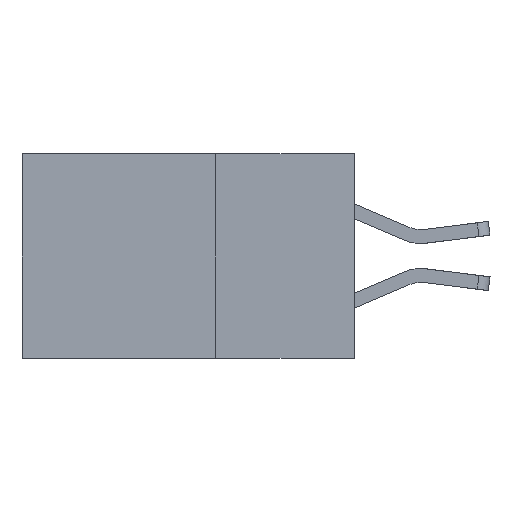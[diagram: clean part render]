
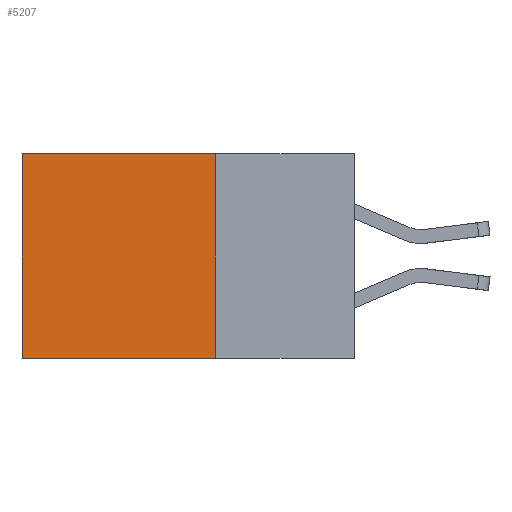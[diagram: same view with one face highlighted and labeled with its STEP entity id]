
A CAD part, left-side view. The second image highlights one B-rep face of the part: STEP entity #5207.
In plain terms, the highlighted planar face has unit normal (-1, 0, 0).
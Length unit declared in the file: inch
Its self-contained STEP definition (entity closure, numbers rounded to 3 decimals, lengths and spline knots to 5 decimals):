
#94 = EDGE_CURVE ( 'NONE', #6212, #6668, #8114, .T. ) ;
#167 = LINE ( 'NONE', #8510, #6126 ) ;
#256 = VERTEX_POINT ( 'NONE', #7802 ) ;
#273 = ORIENTED_EDGE ( 'NONE', *, *, #2507, .T. ) ;
#386 = ORIENTED_EDGE ( 'NONE', *, *, #94, .F. ) ;
#502 = VERTEX_POINT ( 'NONE', #7312 ) ;
#511 = ORIENTED_EDGE ( 'NONE', *, *, #9376, .F. ) ;
#541 = DIRECTION ( 'NONE',  ( 1., 0., 0. ) ) ;
#648 = DIRECTION ( 'NONE',  ( 0., 0., -1. ) ) ;
#697 = CARTESIAN_POINT ( 'NONE',  ( 0.2615, 0.25, -0.37 ) ) ;
#748 = PLANE ( 'NONE',  #6104 ) ;
#918 = VECTOR ( 'NONE', #7294, 39.37008 ) ;
#974 = ORIENTED_EDGE ( 'NONE', *, *, #1633, .T. ) ;
#1185 = LINE ( 'NONE', #9366, #918 ) ;
#1633 = EDGE_CURVE ( 'NONE', #256, #502, #167, .T. ) ;
#1640 = DIRECTION ( 'NONE',  ( 0., 0., -1. ) ) ;
#1772 = EDGE_LOOP ( 'NONE', ( #273, #386, #511, #974 ) ) ;
#2507 = EDGE_CURVE ( 'NONE', #502, #6668, #1185, .T. ) ;
#2547 = CARTESIAN_POINT ( 'NONE',  ( 0.2615, 0.6, -0.37 ) ) ;
#2885 = VECTOR ( 'NONE', #2998, 39.37008 ) ;
#2998 = DIRECTION ( 'NONE',  ( 0., 1., 0. ) ) ;
#5053 = CARTESIAN_POINT ( 'NONE',  ( 0.2615, 0.25, -0.37 ) ) ;
#5207 = ADVANCED_FACE ( 'NONE', ( #9170 ), #748, .F. ) ;
#5712 = DIRECTION ( 'NONE',  ( 0., 1., 0. ) ) ;
#5927 = LINE ( 'NONE', #8103, #9341 ) ;
#6104 = AXIS2_PLACEMENT_3D ( 'NONE', #697, #541, #648 ) ;
#6126 = VECTOR ( 'NONE', #5712, 39.37008 ) ;
#6212 = VERTEX_POINT ( 'NONE', #5053 ) ;
#6668 = VERTEX_POINT ( 'NONE', #2547 ) ;
#7294 = DIRECTION ( 'NONE',  ( 0., 0., -1. ) ) ;
#7312 = CARTESIAN_POINT ( 'NONE',  ( 0.2615, 0.6, 0. ) ) ;
#7549 = CARTESIAN_POINT ( 'NONE',  ( 0.2615, 0.25, -0.37 ) ) ;
#7802 = CARTESIAN_POINT ( 'NONE',  ( 0.2615, 0.25, 0. ) ) ;
#8103 = CARTESIAN_POINT ( 'NONE',  ( 0.2615, 0.25, -0.37 ) ) ;
#8114 = LINE ( 'NONE', #7549, #2885 ) ;
#8510 = CARTESIAN_POINT ( 'NONE',  ( 0.2615, 0.25, 0. ) ) ;
#9170 = FACE_OUTER_BOUND ( 'NONE', #1772, .T. ) ;
#9341 = VECTOR ( 'NONE', #1640, 39.37008 ) ;
#9366 = CARTESIAN_POINT ( 'NONE',  ( 0.2615, 0.6, -0.37 ) ) ;
#9376 = EDGE_CURVE ( 'NONE', #256, #6212, #5927, .T. ) ;
